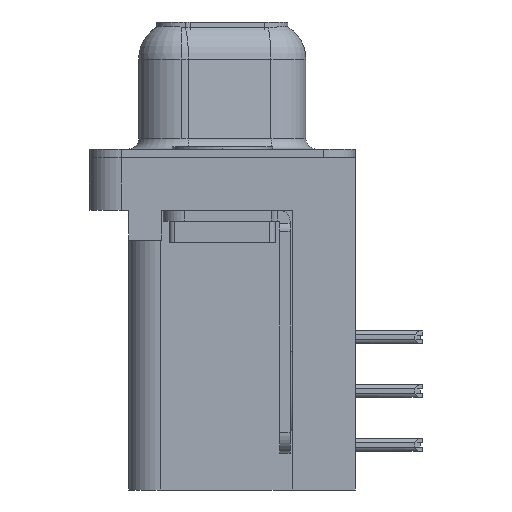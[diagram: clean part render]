
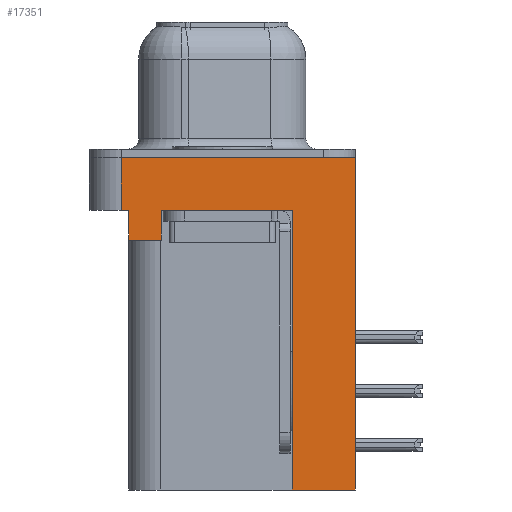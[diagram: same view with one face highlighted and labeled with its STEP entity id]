
A CAD part, left-side view. The second image highlights one B-rep face of the part: STEP entity #17351.
In plain terms, the highlighted planar face has unit normal (-1, 0, 0).
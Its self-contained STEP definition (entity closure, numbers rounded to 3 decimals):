
#451 = EDGE_CURVE ( 'NONE', #35096, #20531, #35544, .T. ) ;
#1162 = EDGE_CURVE ( 'NONE', #14088, #11948, #22305, .T. ) ;
#2141 = EDGE_CURVE ( 'NONE', #35096, #14088, #5768, .T. ) ;
#2648 = DIRECTION ( 'NONE',  ( 0., -1., 0. ) ) ;
#3118 = CARTESIAN_POINT ( 'NONE',  ( -2.935, 4.425, -3.9 ) ) ;
#3150 = EDGE_CURVE ( 'NONE', #35432, #8033, #25659, .T. ) ;
#4418 = EDGE_CURVE ( 'NONE', #35432, #19370, #8297, .T. ) ;
#4686 = VERTEX_POINT ( 'NONE', #18243 ) ;
#4936 = CARTESIAN_POINT ( 'NONE',  ( -2.935, 2.895, -2.5 ) ) ;
#5768 = LINE ( 'NONE', #22143, #6787 ) ;
#6421 = DIRECTION ( 'NONE',  ( 0., 1., 0. ) ) ;
#6787 = VECTOR ( 'NONE', #22189, 1000. ) ;
#7285 = ORIENTED_EDGE ( 'NONE', *, *, #34786, .T. ) ;
#7900 = VECTOR ( 'NONE', #23696, 1000. ) ;
#8033 = VERTEX_POINT ( 'NONE', #29226 ) ;
#8222 = ORIENTED_EDGE ( 'NONE', *, *, #27252, .F. ) ;
#8297 = LINE ( 'NONE', #12221, #7900 ) ;
#9581 = CARTESIAN_POINT ( 'NONE',  ( -2.935, 4.775, -2.5 ) ) ;
#9783 = ORIENTED_EDGE ( 'NONE', *, *, #24085, .F. ) ;
#10018 = CARTESIAN_POINT ( 'NONE',  ( -2.935, 4.425, -3.9 ) ) ;
#10563 = CARTESIAN_POINT ( 'NONE',  ( -2.935, -6.275, -2.5 ) ) ;
#11544 = VERTEX_POINT ( 'NONE', #22845 ) ;
#11570 = LINE ( 'NONE', #9581, #11700 ) ;
#11700 = VECTOR ( 'NONE', #26411, 1000. ) ;
#11948 = VERTEX_POINT ( 'NONE', #16597 ) ;
#12221 = CARTESIAN_POINT ( 'NONE',  ( -2.935, -6.275, -2.5 ) ) ;
#12516 = VECTOR ( 'NONE', #2648, 1000. ) ;
#12753 = LINE ( 'NONE', #19273, #12516 ) ;
#12764 = FACE_OUTER_BOUND ( 'NONE', #26993, .T. ) ;
#13349 = DIRECTION ( 'NONE',  ( -1., 0., 0. ) ) ;
#13872 = DIRECTION ( 'NONE',  ( 0., 0., 1. ) ) ;
#14088 = VERTEX_POINT ( 'NONE', #4936 ) ;
#14285 = ORIENTED_EDGE ( 'NONE', *, *, #4418, .T. ) ;
#15613 = CARTESIAN_POINT ( 'NONE',  ( -2.935, -6.275, -15.7 ) ) ;
#16248 = ORIENTED_EDGE ( 'NONE', *, *, #1162, .T. ) ;
#16597 = CARTESIAN_POINT ( 'NONE',  ( -2.935, -3.295, -2.5 ) ) ;
#16703 = VECTOR ( 'NONE', #34456, 1000. ) ;
#16734 = LINE ( 'NONE', #28732, #16703 ) ;
#17351 = ADVANCED_FACE ( 'NONE', ( #12764 ), #27495, .T. ) ;
#18243 = CARTESIAN_POINT ( 'NONE',  ( -2.935, 4.775, 0. ) ) ;
#18437 = CARTESIAN_POINT ( 'NONE',  ( -2.935, 4.425, -3.9 ) ) ;
#18537 = DIRECTION ( 'NONE',  ( 0., 0., 1. ) ) ;
#19273 = CARTESIAN_POINT ( 'NONE',  ( -2.935, -6.275, -2.5 ) ) ;
#19370 = VERTEX_POINT ( 'NONE', #25772 ) ;
#19846 = DIRECTION ( 'NONE',  ( 0., 1., 0. ) ) ;
#20531 = VERTEX_POINT ( 'NONE', #18437 ) ;
#20877 = CARTESIAN_POINT ( 'NONE',  ( -2.935, -6.275, -2.5 ) ) ;
#21070 = CARTESIAN_POINT ( 'NONE',  ( -2.935, -3.295, -15.7 ) ) ;
#21663 = VECTOR ( 'NONE', #24801, 1000. ) ;
#22143 = CARTESIAN_POINT ( 'NONE',  ( -2.935, 2.895, -3.9 ) ) ;
#22189 = DIRECTION ( 'NONE',  ( 0., 0., 1. ) ) ;
#22305 = LINE ( 'NONE', #20877, #21663 ) ;
#22829 = ORIENTED_EDGE ( 'NONE', *, *, #24774, .F. ) ;
#22845 = CARTESIAN_POINT ( 'NONE',  ( -2.935, 4.775, -2.5 ) ) ;
#23629 = ORIENTED_EDGE ( 'NONE', *, *, #2141, .T. ) ;
#23696 = DIRECTION ( 'NONE',  ( 0., 0., 1. ) ) ;
#24085 = EDGE_CURVE ( 'NONE', #8033, #11948, #29124, .T. ) ;
#24774 = EDGE_CURVE ( 'NONE', #4686, #19370, #16734, .T. ) ;
#24801 = DIRECTION ( 'NONE',  ( 0., -1., 0. ) ) ;
#25329 = VECTOR ( 'NONE', #19846, 1000. ) ;
#25659 = LINE ( 'NONE', #21070, #25329 ) ;
#25772 = CARTESIAN_POINT ( 'NONE',  ( -2.935, -6.275, 0. ) ) ;
#26225 = ORIENTED_EDGE ( 'NONE', *, *, #451, .F. ) ;
#26411 = DIRECTION ( 'NONE',  ( 0., 0., 1. ) ) ;
#26993 = EDGE_LOOP ( 'NONE', ( #22829, #32456, #7285, #8222, #26225, #23629, #16248, #9783, #34265, #14285 ) ) ;
#27252 = EDGE_CURVE ( 'NONE', #20531, #28859, #30524, .T. ) ;
#27495 = PLANE ( 'NONE',  #35519 ) ;
#28032 = CARTESIAN_POINT ( 'NONE',  ( -2.935, 4.425, -2.5 ) ) ;
#28732 = CARTESIAN_POINT ( 'NONE',  ( -2.935, -6.275, 0. ) ) ;
#28859 = VERTEX_POINT ( 'NONE', #28032 ) ;
#29124 = LINE ( 'NONE', #30914, #29431 ) ;
#29226 = CARTESIAN_POINT ( 'NONE',  ( -2.935, -3.295, -15.7 ) ) ;
#29431 = VECTOR ( 'NONE', #13872, 1000. ) ;
#30417 = VECTOR ( 'NONE', #18537, 1000. ) ;
#30524 = LINE ( 'NONE', #10018, #30417 ) ;
#30914 = CARTESIAN_POINT ( 'NONE',  ( -2.935, -3.295, -15.7 ) ) ;
#32456 = ORIENTED_EDGE ( 'NONE', *, *, #34944, .F. ) ;
#33241 = DIRECTION ( 'NONE',  ( 0., 0., 1. ) ) ;
#33993 = CARTESIAN_POINT ( 'NONE',  ( -2.935, 2.895, -3.9 ) ) ;
#34265 = ORIENTED_EDGE ( 'NONE', *, *, #3150, .F. ) ;
#34456 = DIRECTION ( 'NONE',  ( 0., -1., 0. ) ) ;
#34786 = EDGE_CURVE ( 'NONE', #11544, #28859, #12753, .T. ) ;
#34944 = EDGE_CURVE ( 'NONE', #11544, #4686, #11570, .T. ) ;
#35096 = VERTEX_POINT ( 'NONE', #33993 ) ;
#35432 = VERTEX_POINT ( 'NONE', #15613 ) ;
#35519 = AXIS2_PLACEMENT_3D ( 'NONE', #10563, #13349, #33241 ) ;
#35544 = LINE ( 'NONE', #3118, #36035 ) ;
#36035 = VECTOR ( 'NONE', #6421, 1000. ) ;
